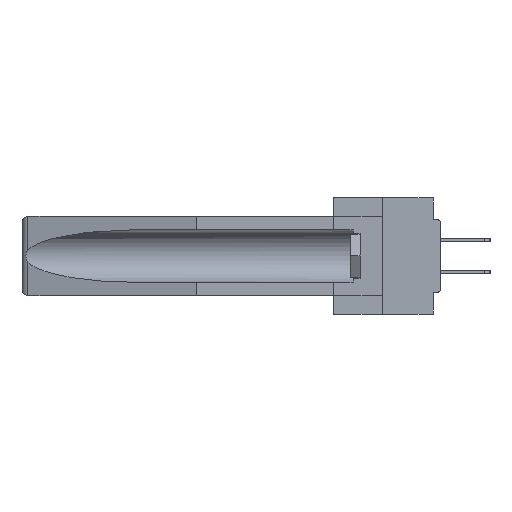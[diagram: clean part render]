
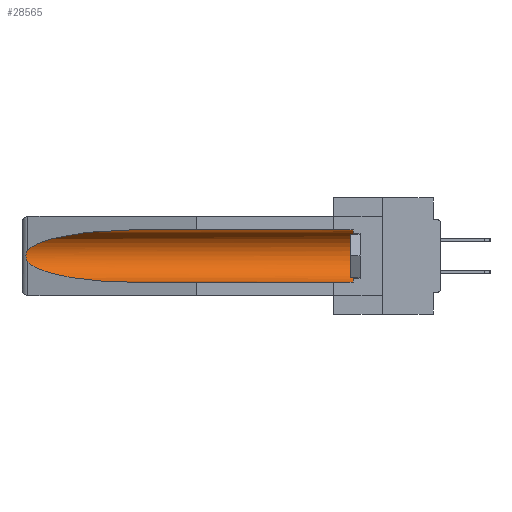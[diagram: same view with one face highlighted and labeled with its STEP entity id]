
A CAD part, left-side view. The second image highlights one B-rep face of the part: STEP entity #28565.
In plain terms, the highlighted cylindrical face has radius 2.857 mm (diameter 5.715 mm), a partial arc.
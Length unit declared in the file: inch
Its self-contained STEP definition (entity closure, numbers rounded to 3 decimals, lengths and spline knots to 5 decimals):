
#859 = VERTEX_POINT ( 'NONE', #28595 ) ;
#947 = VECTOR ( 'NONE', #14557, 39.37008 ) ;
#2245 = CARTESIAN_POINT ( 'NONE',  ( 0.2673, 1.5327, -0.16383 ) ) ;
#2359 = CARTESIAN_POINT ( 'NONE',  ( 0.2675, 1.53308, -0.16763 ) ) ;
#2576 = CARTESIAN_POINT ( 'NONE',  ( 0.2675, 1.53308, -0.17534 ) ) ;
#3256 = CARTESIAN_POINT ( 'NONE',  ( 0.26537, 1.52718, -0.19328 ) ) ;
#3950 = CARTESIAN_POINT ( 'NONE',  ( 0.26537, 1.52718, -0.14972 ) ) ;
#5083 = LINE ( 'NONE', #6819, #12974 ) ;
#5373 = CARTESIAN_POINT ( 'NONE',  ( 0.21114, 1.30732, -0.284 ) ) ;
#6670 = DIRECTION ( 'NONE',  ( 0., -1., 0. ) ) ;
#6819 = CARTESIAN_POINT ( 'NONE',  ( 0.155, -0.30754, -0.059 ) ) ;
#7294 = CARTESIAN_POINT ( 'NONE',  ( 0.155, 0.126, -0.284 ) ) ;
#7524 = ORIENTED_EDGE ( 'NONE', *, *, #8032, .T. ) ;
#7590 = CARTESIAN_POINT ( 'NONE',  ( 0.26654, 1.53092, -0.15636 ) ) ;
#8032 = EDGE_CURVE ( 'NONE', #859, #13260, #13023, .T. ) ;
#8058 = EDGE_CURVE ( 'NONE', #13260, #18965, #14060, .T. ) ;
#8213 = CARTESIAN_POINT ( 'NONE',  ( 0.155, 0.126, -0.059 ) ) ;
#9241 = EDGE_LOOP ( 'NONE', ( #33238, #7524, #15294, #16415, #25907, #32068 ) ) ;
#10355 = CARTESIAN_POINT ( 'NONE',  ( 0.2673, 1.53269, -0.17917 ) ) ;
#10570 = CARTESIAN_POINT ( 'NONE',  ( 0.25451, 1.48313, -0.24835 ) ) ;
#12695 = CARTESIAN_POINT ( 'NONE',  ( 0.26597, 1.5296, -0.19026 ) ) ;
#12974 = VECTOR ( 'NONE', #33623, 39.37008 ) ;
#13023 = B_SPLINE_CURVE_WITH_KNOTS ( 'NONE', 3,
 ( #18296, #23516, #7590, #2245, #2359, #2576, #10355, #26492, #12695, #15368 ),
 .UNSPECIFIED., .F., .F.,
 ( 4, 2, 2, 2, 4 ),
 ( 0., 0.00029, 0.00058, 0.00087, 0.00117 ),
 .UNSPECIFIED. ) ;
#13260 = VERTEX_POINT ( 'NONE', #3256 ) ;
#14060 =( BOUNDED_CURVE ( )  B_SPLINE_CURVE ( 3, ( #16148, #10570, #5373, #21445 ),
 .UNSPECIFIED., .F., .F. ) 
 B_SPLINE_CURVE_WITH_KNOTS ( ( 4, 4 ),
 ( 0.1948, 1.5708 ),
 .UNSPECIFIED. ) 
 CURVE ( )  GEOMETRIC_REPRESENTATION_ITEM ( )  RATIONAL_B_SPLINE_CURVE ( ( 1., 0.848, 0.848, 1. ) ) 
 REPRESENTATION_ITEM ( '' )  );
#14134 = CARTESIAN_POINT ( 'NONE',  ( 0.155, 1.07973, -0.284 ) ) ;
#14557 = DIRECTION ( 'NONE',  ( 0., 1., 0. ) ) ;
#15294 = ORIENTED_EDGE ( 'NONE', *, *, #8058, .T. ) ;
#15368 = CARTESIAN_POINT ( 'NONE',  ( 0.26537, 1.52718, -0.19328 ) ) ;
#15793 = VERTEX_POINT ( 'NONE', #7294 ) ;
#16148 = CARTESIAN_POINT ( 'NONE',  ( 0.26537, 1.52718, -0.19328 ) ) ;
#16415 = ORIENTED_EDGE ( 'NONE', *, *, #33151, .F. ) ;
#17823 = AXIS2_PLACEMENT_3D ( 'NONE', #29062, #29282, #24180 ) ;
#18296 = CARTESIAN_POINT ( 'NONE',  ( 0.26537, 1.52718, -0.14972 ) ) ;
#18309 = CIRCLE ( 'NONE', #32739, 0.1125 ) ;
#18965 = VERTEX_POINT ( 'NONE', #14134 ) ;
#19906 = CARTESIAN_POINT ( 'NONE',  ( 0.21114, 1.30732, -0.059 ) ) ;
#21445 = CARTESIAN_POINT ( 'NONE',  ( 0.155, 1.07973, -0.284 ) ) ;
#21965 = EDGE_CURVE ( 'NONE', #32684, #859, #22835, .T. ) ;
#22496 = DIRECTION ( 'NONE',  ( 0., 0., 1. ) ) ;
#22835 =( BOUNDED_CURVE ( )  B_SPLINE_CURVE ( 3, ( #27740, #19906, #25428, #3950 ),
 .UNSPECIFIED., .F., .F. ) 
 B_SPLINE_CURVE_WITH_KNOTS ( ( 4, 4 ),
 ( 4.71239, 6.08839 ),
 .UNSPECIFIED. ) 
 CURVE ( )  GEOMETRIC_REPRESENTATION_ITEM ( )  RATIONAL_B_SPLINE_CURVE ( ( 1., 0.848, 0.848, 1. ) ) 
 REPRESENTATION_ITEM ( '' )  );
#23327 = FACE_OUTER_BOUND ( 'NONE', #9241, .T. ) ;
#23516 = CARTESIAN_POINT ( 'NONE',  ( 0.26597, 1.52961, -0.15275 ) ) ;
#23699 = EDGE_CURVE ( 'NONE', #15793, #31311, #18309, .T. ) ;
#24180 = DIRECTION ( 'NONE',  ( 0., 0., 1. ) ) ;
#25428 = CARTESIAN_POINT ( 'NONE',  ( 0.25451, 1.48313, -0.09465 ) ) ;
#25907 = ORIENTED_EDGE ( 'NONE', *, *, #23699, .T. ) ;
#26492 = CARTESIAN_POINT ( 'NONE',  ( 0.26655, 1.53094, -0.18657 ) ) ;
#27740 = CARTESIAN_POINT ( 'NONE',  ( 0.155, 1.07973, -0.059 ) ) ;
#27919 = EDGE_CURVE ( 'NONE', #31311, #32684, #5083, .T. ) ;
#28223 = CARTESIAN_POINT ( 'NONE',  ( 0.155, -0.30754, -0.284 ) ) ;
#28565 = ADVANCED_FACE ( 'NONE', ( #23327 ), #31972, .F. ) ;
#28595 = CARTESIAN_POINT ( 'NONE',  ( 0.26537, 1.52718, -0.14972 ) ) ;
#29062 = CARTESIAN_POINT ( 'NONE',  ( 0.155, -0.30754, -0.1715 ) ) ;
#29282 = DIRECTION ( 'NONE',  ( 0., 1., 0. ) ) ;
#31311 = VERTEX_POINT ( 'NONE', #8213 ) ;
#31897 = CARTESIAN_POINT ( 'NONE',  ( 0.155, 1.07973, -0.059 ) ) ;
#31972 = CYLINDRICAL_SURFACE ( 'NONE', #17823, 0.1125 ) ;
#32068 = ORIENTED_EDGE ( 'NONE', *, *, #27919, .T. ) ;
#32482 = LINE ( 'NONE', #28223, #947 ) ;
#32684 = VERTEX_POINT ( 'NONE', #31897 ) ;
#32739 = AXIS2_PLACEMENT_3D ( 'NONE', #33106, #6670, #22496 ) ;
#33106 = CARTESIAN_POINT ( 'NONE',  ( 0.155, 0.126, -0.1715 ) ) ;
#33151 = EDGE_CURVE ( 'NONE', #15793, #18965, #32482, .T. ) ;
#33238 = ORIENTED_EDGE ( 'NONE', *, *, #21965, .T. ) ;
#33623 = DIRECTION ( 'NONE',  ( 0., 1., 0. ) ) ;
